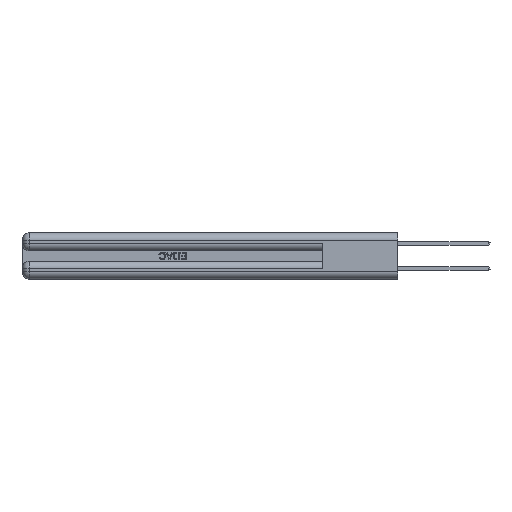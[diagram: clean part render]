
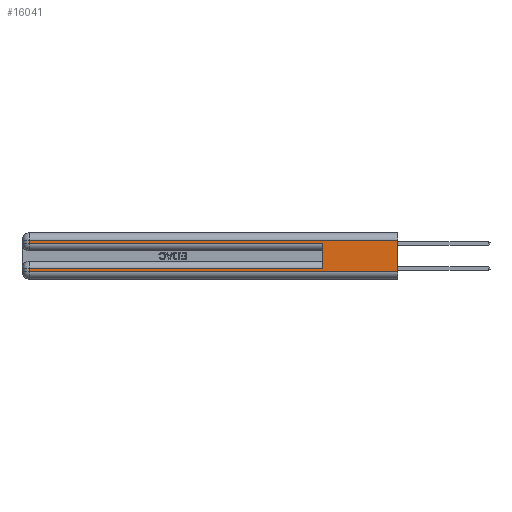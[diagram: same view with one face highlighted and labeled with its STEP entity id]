
A CAD part, left-side view. The second image highlights one B-rep face of the part: STEP entity #16041.
In plain terms, the highlighted planar face has unit normal (-1, 0, 0).
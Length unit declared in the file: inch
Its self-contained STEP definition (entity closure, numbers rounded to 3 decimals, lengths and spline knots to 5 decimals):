
#1822 = LINE ( 'NONE', #13192, #21882 ) ;
#2430 = LINE ( 'NONE', #43923, #11852 ) ;
#2671 = CARTESIAN_POINT ( 'NONE',  ( 0., 0., 0.06 ) ) ;
#2701 = VERTEX_POINT ( 'NONE', #2671 ) ;
#3516 = PLANE ( 'NONE',  #45870 ) ;
#4429 = VERTEX_POINT ( 'NONE', #17922 ) ;
#4534 = ORIENTED_EDGE ( 'NONE', *, *, #31211, .T. ) ;
#4898 = CARTESIAN_POINT ( 'NONE',  ( 0., 0.6, 0.285 ) ) ;
#6383 = VECTOR ( 'NONE', #36114, 39.37008 ) ;
#7591 = VECTOR ( 'NONE', #26951, 39.37008 ) ;
#8375 = EDGE_CURVE ( 'NONE', #41142, #34739, #1822, .T. ) ;
#8887 = CARTESIAN_POINT ( 'NONE',  ( 0., 0., 0.31 ) ) ;
#9058 = ORIENTED_EDGE ( 'NONE', *, *, #48249, .T. ) ;
#10260 = VECTOR ( 'NONE', #34275, 39.37008 ) ;
#11092 = VERTEX_POINT ( 'NONE', #17815 ) ;
#11578 = DIRECTION ( 'NONE',  ( 0., 0., -1. ) ) ;
#11852 = VECTOR ( 'NONE', #12099, 39.37008 ) ;
#12099 = DIRECTION ( 'NONE',  ( 0., 0., 1. ) ) ;
#13192 = CARTESIAN_POINT ( 'NONE',  ( 0., 0., 0.31 ) ) ;
#14642 = EDGE_LOOP ( 'NONE', ( #44698, #27168, #9058, #30176, #37465, #21244, #42989, #4534 ) ) ;
#16041 = ADVANCED_FACE ( 'NONE', ( #36377 ), #3516, .F. ) ;
#17187 = DIRECTION ( 'NONE',  ( 0., 1., 0. ) ) ;
#17353 = VECTOR ( 'NONE', #19589, 39.37008 ) ;
#17815 = CARTESIAN_POINT ( 'NONE',  ( 0., 2.94, 0.085 ) ) ;
#17922 = CARTESIAN_POINT ( 'NONE',  ( 0., 2.94, 0.06 ) ) ;
#19287 = VERTEX_POINT ( 'NONE', #28592 ) ;
#19589 = DIRECTION ( 'NONE',  ( 0., 1., 0. ) ) ;
#20902 = LINE ( 'NONE', #38130, #10260 ) ;
#21244 = ORIENTED_EDGE ( 'NONE', *, *, #24536, .T. ) ;
#21882 = VECTOR ( 'NONE', #17187, 39.37008 ) ;
#22470 = CARTESIAN_POINT ( 'NONE',  ( 0., 0., 0.37 ) ) ;
#23414 = CARTESIAN_POINT ( 'NONE',  ( 0., 0., 0.085 ) ) ;
#24018 = CARTESIAN_POINT ( 'NONE',  ( 0., 0., 0.06 ) ) ;
#24536 = EDGE_CURVE ( 'NONE', #42734, #11092, #49272, .T. ) ;
#25625 = CARTESIAN_POINT ( 'NONE',  ( 0., 0., 0.285 ) ) ;
#26951 = DIRECTION ( 'NONE',  ( 0., 0., -1. ) ) ;
#27031 = LINE ( 'NONE', #22470, #37665 ) ;
#27168 = ORIENTED_EDGE ( 'NONE', *, *, #8375, .T. ) ;
#27765 = EDGE_CURVE ( 'NONE', #19287, #36486, #29596, .T. ) ;
#28592 = CARTESIAN_POINT ( 'NONE',  ( 0., 2.94, 0.285 ) ) ;
#29596 = LINE ( 'NONE', #25625, #49628 ) ;
#29641 = DIRECTION ( 'NONE',  ( 0., -1., 0. ) ) ;
#30120 = LINE ( 'NONE', #46921, #7591 ) ;
#30176 = ORIENTED_EDGE ( 'NONE', *, *, #27765, .T. ) ;
#30203 = EDGE_CURVE ( 'NONE', #11092, #4429, #20902, .T. ) ;
#31211 = EDGE_CURVE ( 'NONE', #4429, #2701, #37072, .T. ) ;
#31482 = CARTESIAN_POINT ( 'NONE',  ( 0., 0., 0.37 ) ) ;
#34275 = DIRECTION ( 'NONE',  ( 0., 0., -1. ) ) ;
#34739 = VERTEX_POINT ( 'NONE', #36734 ) ;
#35530 = DIRECTION ( 'NONE',  ( 1., 0., 0. ) ) ;
#36114 = DIRECTION ( 'NONE',  ( 0., -1., 0. ) ) ;
#36377 = FACE_OUTER_BOUND ( 'NONE', #14642, .T. ) ;
#36486 = VERTEX_POINT ( 'NONE', #4898 ) ;
#36734 = CARTESIAN_POINT ( 'NONE',  ( 0., 2.94, 0.31 ) ) ;
#37072 = LINE ( 'NONE', #24018, #6383 ) ;
#37298 = EDGE_CURVE ( 'NONE', #41142, #2701, #27031, .T. ) ;
#37465 = ORIENTED_EDGE ( 'NONE', *, *, #46016, .F. ) ;
#37665 = VECTOR ( 'NONE', #42428, 39.37008 ) ;
#38130 = CARTESIAN_POINT ( 'NONE',  ( 0., 2.94, 0.37 ) ) ;
#38525 = CARTESIAN_POINT ( 'NONE',  ( 0., 0.6, 0.085 ) ) ;
#41142 = VERTEX_POINT ( 'NONE', #8887 ) ;
#42428 = DIRECTION ( 'NONE',  ( 0., 0., -1. ) ) ;
#42734 = VERTEX_POINT ( 'NONE', #38525 ) ;
#42989 = ORIENTED_EDGE ( 'NONE', *, *, #30203, .T. ) ;
#43923 = CARTESIAN_POINT ( 'NONE',  ( 0., 0.6, 0.145 ) ) ;
#44698 = ORIENTED_EDGE ( 'NONE', *, *, #37298, .F. ) ;
#45870 = AXIS2_PLACEMENT_3D ( 'NONE', #31482, #35530, #11578 ) ;
#46016 = EDGE_CURVE ( 'NONE', #42734, #36486, #2430, .T. ) ;
#46921 = CARTESIAN_POINT ( 'NONE',  ( 0., 2.94, 0.37 ) ) ;
#48249 = EDGE_CURVE ( 'NONE', #34739, #19287, #30120, .T. ) ;
#49272 = LINE ( 'NONE', #23414, #17353 ) ;
#49628 = VECTOR ( 'NONE', #29641, 39.37008 ) ;
